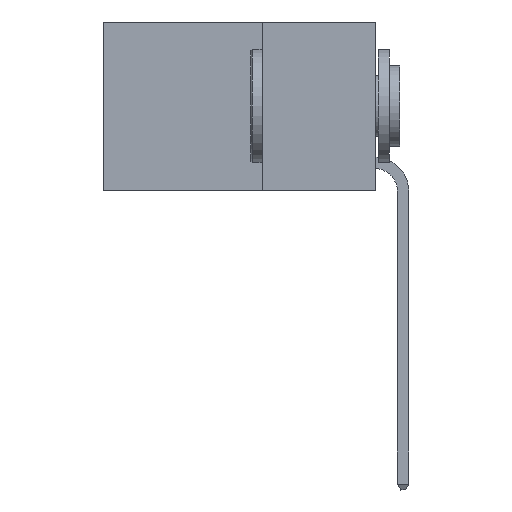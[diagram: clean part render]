
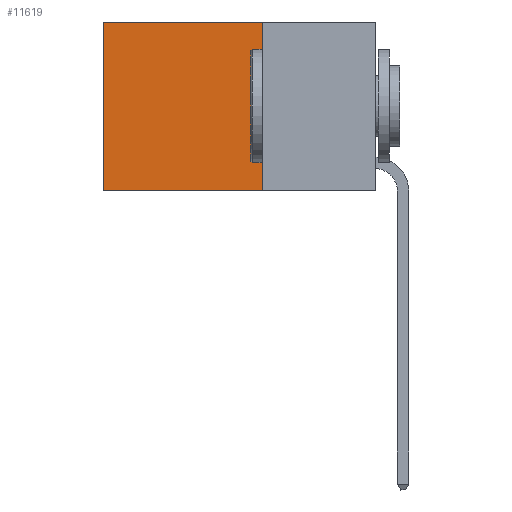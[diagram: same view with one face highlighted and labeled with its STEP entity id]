
A CAD part, left-side view. The second image highlights one B-rep face of the part: STEP entity #11619.
In plain terms, the highlighted planar face has unit normal (-1, 0, 0).
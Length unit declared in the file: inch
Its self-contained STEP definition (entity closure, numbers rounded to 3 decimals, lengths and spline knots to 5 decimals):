
#836 = VECTOR ( 'NONE', #1221, 39.37008 ) ;
#1026 = EDGE_CURVE ( 'NONE', #2503, #16222, #16922, .T. ) ;
#1129 = DIRECTION ( 'NONE',  ( 0., 0., -1. ) ) ;
#1221 = DIRECTION ( 'NONE',  ( 0., 0., -1. ) ) ;
#2358 = VERTEX_POINT ( 'NONE', #6268 ) ;
#2503 = VERTEX_POINT ( 'NONE', #2565 ) ;
#2558 = DIRECTION ( 'NONE',  ( 1., 0., 0. ) ) ;
#2565 = CARTESIAN_POINT ( 'NONE',  ( 0.2625, 0.6, 0. ) ) ;
#2949 = CARTESIAN_POINT ( 'NONE',  ( 0.2625, 0.25, 0. ) ) ;
#3743 = LINE ( 'NONE', #19586, #12299 ) ;
#3889 = CARTESIAN_POINT ( 'NONE',  ( 0.2625, 0.25, 0. ) ) ;
#4391 = VECTOR ( 'NONE', #18491, 39.37008 ) ;
#4812 = EDGE_CURVE ( 'NONE', #9851, #2503, #16924, .T. ) ;
#4907 = ORIENTED_EDGE ( 'NONE', *, *, #4812, .T. ) ;
#5215 = EDGE_LOOP ( 'NONE', ( #9605, #15743, #6463, #4907 ) ) ;
#6268 = CARTESIAN_POINT ( 'NONE',  ( 0.2625, 0.25, -0.37 ) ) ;
#6463 = ORIENTED_EDGE ( 'NONE', *, *, #14324, .F. ) ;
#7060 = FACE_OUTER_BOUND ( 'NONE', #5215, .T. ) ;
#8928 = CARTESIAN_POINT ( 'NONE',  ( 0.2625, 0.25, 0. ) ) ;
#9230 = DIRECTION ( 'NONE',  ( 0., 1., 0. ) ) ;
#9605 = ORIENTED_EDGE ( 'NONE', *, *, #1026, .T. ) ;
#9851 = VERTEX_POINT ( 'NONE', #16505 ) ;
#10267 = PLANE ( 'NONE',  #10983 ) ;
#10983 = AXIS2_PLACEMENT_3D ( 'NONE', #8928, #2558, #1129 ) ;
#11619 = ADVANCED_FACE ( 'NONE', ( #7060 ), #10267, .F. ) ;
#11774 = DIRECTION ( 'NONE',  ( 0., 1., 0. ) ) ;
#12284 = EDGE_CURVE ( 'NONE', #2358, #16222, #3743, .T. ) ;
#12299 = VECTOR ( 'NONE', #11774, 39.37008 ) ;
#13284 = CARTESIAN_POINT ( 'NONE',  ( 0.2625, 0.6, -0.37 ) ) ;
#14324 = EDGE_CURVE ( 'NONE', #9851, #2358, #15125, .T. ) ;
#15125 = LINE ( 'NONE', #3889, #4391 ) ;
#15743 = ORIENTED_EDGE ( 'NONE', *, *, #12284, .F. ) ;
#16222 = VERTEX_POINT ( 'NONE', #13284 ) ;
#16505 = CARTESIAN_POINT ( 'NONE',  ( 0.2625, 0.25, 0. ) ) ;
#16922 = LINE ( 'NONE', #19621, #836 ) ;
#16924 = LINE ( 'NONE', #2949, #19156 ) ;
#18491 = DIRECTION ( 'NONE',  ( 0., 0., -1. ) ) ;
#19156 = VECTOR ( 'NONE', #9230, 39.37008 ) ;
#19586 = CARTESIAN_POINT ( 'NONE',  ( 0.2625, 0.25, -0.37 ) ) ;
#19621 = CARTESIAN_POINT ( 'NONE',  ( 0.2625, 0.6, 0. ) ) ;
